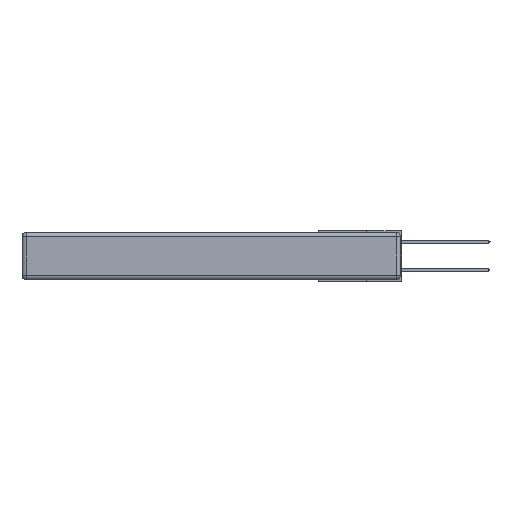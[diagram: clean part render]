
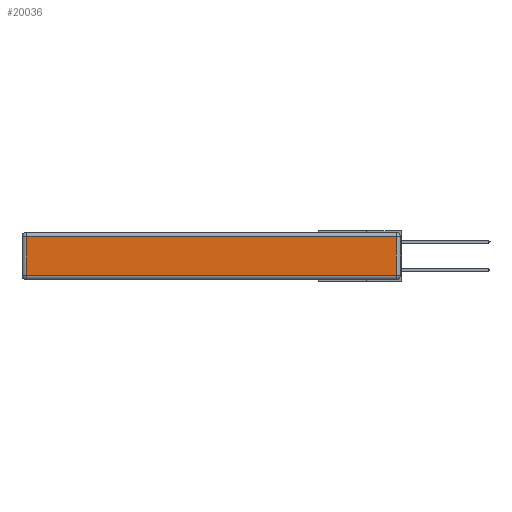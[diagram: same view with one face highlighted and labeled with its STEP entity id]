
A CAD part, left-side view. The second image highlights one B-rep face of the part: STEP entity #20036.
In plain terms, the highlighted planar face has unit normal (-1, 0, 0).
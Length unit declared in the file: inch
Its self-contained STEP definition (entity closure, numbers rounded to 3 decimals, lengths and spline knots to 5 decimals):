
#780 = LINE ( 'NONE', #21973, #20764 ) ;
#1775 = VECTOR ( 'NONE', #13430, 39.37008 ) ;
#3865 = ORIENTED_EDGE ( 'NONE', *, *, #24939, .T. ) ;
#5164 = DIRECTION ( 'NONE',  ( -1., 0., 0. ) ) ;
#6445 = DIRECTION ( 'NONE',  ( 0., 1., 0. ) ) ;
#6967 = DIRECTION ( 'NONE',  ( 0., -1., 0. ) ) ;
#8844 = CARTESIAN_POINT ( 'NONE',  ( 0., 0., -0.313 ) ) ;
#9618 = VECTOR ( 'NONE', #22523, 39.37008 ) ;
#10935 = DIRECTION ( 'NONE',  ( 0., 0., 1. ) ) ;
#11105 = PLANE ( 'NONE',  #20779 ) ;
#13430 = DIRECTION ( 'NONE',  ( 0., 0., -1. ) ) ;
#13920 = CARTESIAN_POINT ( 'NONE',  ( 0., 0.03, -0.03 ) ) ;
#14794 = LINE ( 'NONE', #20603, #9618 ) ;
#15564 = CARTESIAN_POINT ( 'NONE',  ( 0., 0.03, -0.313 ) ) ;
#15921 = VERTEX_POINT ( 'NONE', #16805 ) ;
#16022 = EDGE_CURVE ( 'NONE', #15921, #17065, #24943, .T. ) ;
#16805 = CARTESIAN_POINT ( 'NONE',  ( 0., 2.72, -0.313 ) ) ;
#16813 = VECTOR ( 'NONE', #6967, 39.37008 ) ;
#16845 = LINE ( 'NONE', #17106, #1775 ) ;
#17065 = VERTEX_POINT ( 'NONE', #15564 ) ;
#17084 = ORIENTED_EDGE ( 'NONE', *, *, #16022, .T. ) ;
#17106 = CARTESIAN_POINT ( 'NONE',  ( 0., 2.72, -0.343 ) ) ;
#18664 = CARTESIAN_POINT ( 'NONE',  ( 0., 2.72, -0.03 ) ) ;
#18852 = CARTESIAN_POINT ( 'NONE',  ( 0., 0., -0.343 ) ) ;
#20036 = ADVANCED_FACE ( 'NONE', ( #20518 ), #11105, .T. ) ;
#20353 = EDGE_CURVE ( 'NONE', #17065, #21276, #14794, .T. ) ;
#20518 = FACE_OUTER_BOUND ( 'NONE', #22793, .T. ) ;
#20603 = CARTESIAN_POINT ( 'NONE',  ( 0., 0.03, -0.343 ) ) ;
#20764 = VECTOR ( 'NONE', #6445, 39.37008 ) ;
#20779 = AXIS2_PLACEMENT_3D ( 'NONE', #18852, #5164, #10935 ) ;
#21276 = VERTEX_POINT ( 'NONE', #13920 ) ;
#21454 = EDGE_CURVE ( 'NONE', #21276, #22309, #780, .T. ) ;
#21973 = CARTESIAN_POINT ( 'NONE',  ( 0., 2.75, -0.03 ) ) ;
#22279 = ORIENTED_EDGE ( 'NONE', *, *, #21454, .T. ) ;
#22309 = VERTEX_POINT ( 'NONE', #18664 ) ;
#22523 = DIRECTION ( 'NONE',  ( 0., 0., 1. ) ) ;
#22793 = EDGE_LOOP ( 'NONE', ( #17084, #24710, #22279, #3865 ) ) ;
#24710 = ORIENTED_EDGE ( 'NONE', *, *, #20353, .T. ) ;
#24939 = EDGE_CURVE ( 'NONE', #22309, #15921, #16845, .T. ) ;
#24943 = LINE ( 'NONE', #8844, #16813 ) ;
